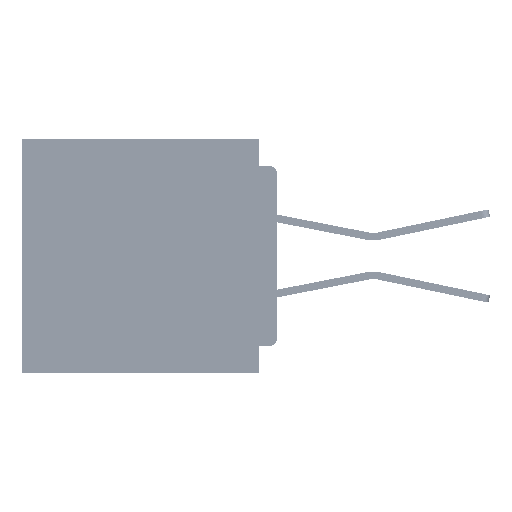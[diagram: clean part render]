
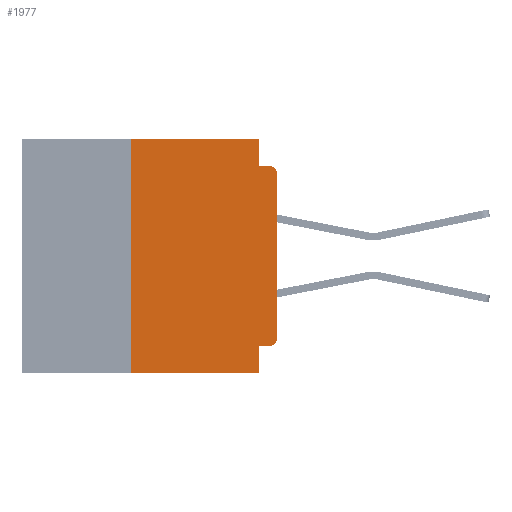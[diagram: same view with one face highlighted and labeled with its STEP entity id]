
A CAD part, left-side view. The second image highlights one B-rep face of the part: STEP entity #1977.
In plain terms, the highlighted planar face has unit normal (-1, 0, 0).
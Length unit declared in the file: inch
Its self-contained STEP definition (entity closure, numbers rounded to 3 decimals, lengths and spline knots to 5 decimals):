
#46 = CARTESIAN_POINT ( 'NONE',  ( 0., 0.031, -0.4 ) ) ;
#47 = ORIENTED_EDGE ( 'NONE', *, *, #46344, .F. ) ;
#281 = DIRECTION ( 'NONE',  ( 0., 0., -1. ) ) ;
#621 = CARTESIAN_POINT ( 'NONE',  ( 0., 0.031, -0.045 ) ) ;
#695 = AXIS2_PLACEMENT_3D ( 'NONE', #51614, #51056, #50889 ) ;
#1977 = ADVANCED_FACE ( 'NONE', ( #14587 ), #51211, .F. ) ;
#2006 = CARTESIAN_POINT ( 'NONE',  ( 0., 0.437, 0. ) ) ;
#2274 = EDGE_CURVE ( 'NONE', #33863, #16322, #13737, .T. ) ;
#2418 = LINE ( 'NONE', #2006, #15175 ) ;
#3860 = ORIENTED_EDGE ( 'NONE', *, *, #2274, .T. ) ;
#4670 = CARTESIAN_POINT ( 'NONE',  ( 0., 0.031, -0.4 ) ) ;
#6385 = EDGE_CURVE ( 'NONE', #8506, #31130, #58219, .T. ) ;
#7656 = AXIS2_PLACEMENT_3D ( 'NONE', #13933, #51977, #19379 ) ;
#7775 = CARTESIAN_POINT ( 'NONE',  ( 0., 0., -0.355 ) ) ;
#8506 = VERTEX_POINT ( 'NONE', #31134 ) ;
#9007 = EDGE_CURVE ( 'NONE', #17374, #65225, #39256, .T. ) ;
#9182 = CARTESIAN_POINT ( 'NONE',  ( 0., 0.25, -0.4 ) ) ;
#9508 = CARTESIAN_POINT ( 'NONE',  ( 0., 0., -0.34 ) ) ;
#9600 = ORIENTED_EDGE ( 'NONE', *, *, #64387, .F. ) ;
#10324 = VECTOR ( 'NONE', #67773, 39.37008 ) ;
#11030 = ORIENTED_EDGE ( 'NONE', *, *, #6385, .F. ) ;
#11500 = ORIENTED_EDGE ( 'NONE', *, *, #68022, .F. ) ;
#13414 = ORIENTED_EDGE ( 'NONE', *, *, #20598, .T. ) ;
#13737 = LINE ( 'NONE', #39917, #53697 ) ;
#13933 = CARTESIAN_POINT ( 'NONE',  ( 0., 0.015, -0.06 ) ) ;
#14163 = DIRECTION ( 'NONE',  ( -1., 0., 0. ) ) ;
#14263 = CARTESIAN_POINT ( 'NONE',  ( 0., 0.031, -0.355 ) ) ;
#14587 = FACE_OUTER_BOUND ( 'NONE', #28047, .T. ) ;
#15175 = VECTOR ( 'NONE', #18419, 39.37008 ) ;
#15334 = VECTOR ( 'NONE', #25077, 39.37008 ) ;
#16018 = CARTESIAN_POINT ( 'NONE',  ( 0., 0., -0.045 ) ) ;
#16322 = VERTEX_POINT ( 'NONE', #63303 ) ;
#17188 = LINE ( 'NONE', #16018, #57092 ) ;
#17374 = VERTEX_POINT ( 'NONE', #50987 ) ;
#18080 = DIRECTION ( 'NONE',  ( 0., 0., -1. ) ) ;
#18419 = DIRECTION ( 'NONE',  ( 0., -1., 0. ) ) ;
#19379 = DIRECTION ( 'NONE',  ( 0., 0., -1. ) ) ;
#20510 = LINE ( 'NONE', #50536, #49477 ) ;
#20598 = EDGE_CURVE ( 'NONE', #49889, #22975, #20510, .T. ) ;
#22597 = VERTEX_POINT ( 'NONE', #44930 ) ;
#22798 = LINE ( 'NONE', #46, #64323 ) ;
#22975 = VERTEX_POINT ( 'NONE', #4670 ) ;
#25077 = DIRECTION ( 'NONE',  ( 0., 0., 1. ) ) ;
#25304 = CIRCLE ( 'NONE', #7656, 0.015 ) ;
#25868 = AXIS2_PLACEMENT_3D ( 'NONE', #46753, #14163, #52197 ) ;
#28047 = EDGE_LOOP ( 'NONE', ( #3860, #44418, #11500, #11030, #9600, #67490, #13414, #47, #34078, #43596 ) ) ;
#29445 = EDGE_CURVE ( 'NONE', #49889, #63925, #31521, .T. ) ;
#31079 = VECTOR ( 'NONE', #18080, 39.37008 ) ;
#31130 = VERTEX_POINT ( 'NONE', #621 ) ;
#31134 = CARTESIAN_POINT ( 'NONE',  ( 0., 0.031, 0. ) ) ;
#31521 = LINE ( 'NONE', #57371, #15334 ) ;
#32481 = DIRECTION ( 'NONE',  ( 0., -1., 0. ) ) ;
#33863 = VERTEX_POINT ( 'NONE', #9508 ) ;
#34078 = ORIENTED_EDGE ( 'NONE', *, *, #9007, .F. ) ;
#39200 = DIRECTION ( 'NONE',  ( 0., 0., 1. ) ) ;
#39256 = LINE ( 'NONE', #7775, #10324 ) ;
#39917 = CARTESIAN_POINT ( 'NONE',  ( 0., 0., 0. ) ) ;
#43596 = ORIENTED_EDGE ( 'NONE', *, *, #58003, .T. ) ;
#44418 = ORIENTED_EDGE ( 'NONE', *, *, #57971, .T. ) ;
#44930 = CARTESIAN_POINT ( 'NONE',  ( 0., 0.015, -0.045 ) ) ;
#46344 = EDGE_CURVE ( 'NONE', #65225, #22975, #22798, .T. ) ;
#46753 = CARTESIAN_POINT ( 'NONE',  ( 0., 0.015, -0.34 ) ) ;
#49477 = VECTOR ( 'NONE', #66783, 39.37008 ) ;
#49889 = VERTEX_POINT ( 'NONE', #9182 ) ;
#50536 = CARTESIAN_POINT ( 'NONE',  ( 0., 0.437, -0.4 ) ) ;
#50666 = CARTESIAN_POINT ( 'NONE',  ( 0., 0.031, 0. ) ) ;
#50889 = DIRECTION ( 'NONE',  ( 0., 0., -1. ) ) ;
#50987 = CARTESIAN_POINT ( 'NONE',  ( 0., 0.015, -0.355 ) ) ;
#51056 = DIRECTION ( 'NONE',  ( 1., 0., 0. ) ) ;
#51211 = PLANE ( 'NONE',  #695 ) ;
#51614 = CARTESIAN_POINT ( 'NONE',  ( 0., 0.437, 0. ) ) ;
#51977 = DIRECTION ( 'NONE',  ( -1., 0., 0. ) ) ;
#52197 = DIRECTION ( 'NONE',  ( 0., 0., -1. ) ) ;
#52527 = CIRCLE ( 'NONE', #25868, 0.015 ) ;
#53697 = VECTOR ( 'NONE', #39200, 39.37008 ) ;
#56791 = CARTESIAN_POINT ( 'NONE',  ( 0., 0.25, 0. ) ) ;
#57092 = VECTOR ( 'NONE', #32481, 39.37008 ) ;
#57371 = CARTESIAN_POINT ( 'NONE',  ( 0., 0.25, -0.4 ) ) ;
#57971 = EDGE_CURVE ( 'NONE', #16322, #22597, #25304, .T. ) ;
#58003 = EDGE_CURVE ( 'NONE', #17374, #33863, #52527, .T. ) ;
#58219 = LINE ( 'NONE', #50666, #31079 ) ;
#63303 = CARTESIAN_POINT ( 'NONE',  ( 0., 0., -0.06 ) ) ;
#63925 = VERTEX_POINT ( 'NONE', #56791 ) ;
#64323 = VECTOR ( 'NONE', #281, 39.37008 ) ;
#64387 = EDGE_CURVE ( 'NONE', #63925, #8506, #2418, .T. ) ;
#65225 = VERTEX_POINT ( 'NONE', #14263 ) ;
#66783 = DIRECTION ( 'NONE',  ( 0., -1., 0. ) ) ;
#67490 = ORIENTED_EDGE ( 'NONE', *, *, #29445, .F. ) ;
#67773 = DIRECTION ( 'NONE',  ( 0., 1., 0. ) ) ;
#68022 = EDGE_CURVE ( 'NONE', #31130, #22597, #17188, .T. ) ;
